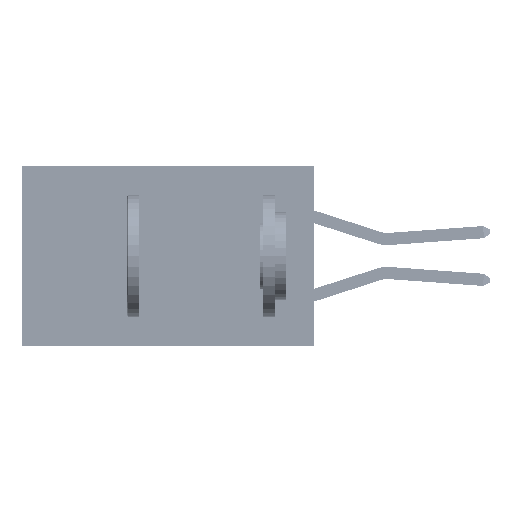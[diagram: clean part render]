
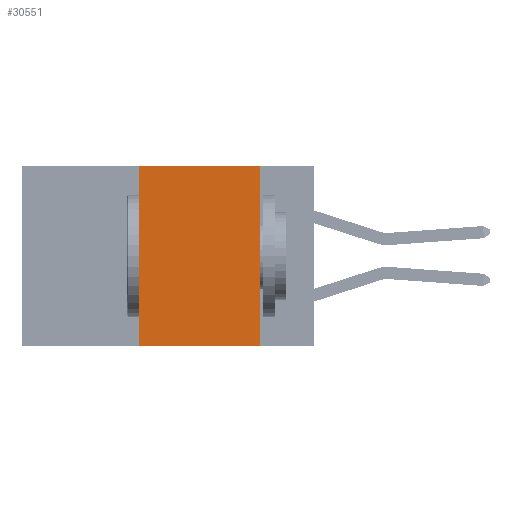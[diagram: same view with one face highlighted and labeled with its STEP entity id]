
A CAD part, left-side view. The second image highlights one B-rep face of the part: STEP entity #30551.
In plain terms, the highlighted planar face has unit normal (-1, 0, 0).
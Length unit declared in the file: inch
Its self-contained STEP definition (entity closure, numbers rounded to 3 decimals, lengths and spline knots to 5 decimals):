
#1260 = VECTOR ( 'NONE', #45532, 39.37008 ) ;
#5038 = CARTESIAN_POINT ( 'NONE',  ( 0., 0.11, 0. ) ) ;
#5152 = ORIENTED_EDGE ( 'NONE', *, *, #28392, .F. ) ;
#5831 = ORIENTED_EDGE ( 'NONE', *, *, #29548, .F. ) ;
#6584 = VECTOR ( 'NONE', #47407, 39.37008 ) ;
#8929 = CARTESIAN_POINT ( 'NONE',  ( 0., 0.36, 0. ) ) ;
#11701 = VERTEX_POINT ( 'NONE', #17921 ) ;
#12452 = EDGE_LOOP ( 'NONE', ( #28630, #5152, #5831, #37780 ) ) ;
#14722 = FACE_OUTER_BOUND ( 'NONE', #12452, .T. ) ;
#15521 = CARTESIAN_POINT ( 'NONE',  ( 0., 0.6, -0.37 ) ) ;
#16817 = LINE ( 'NONE', #29601, #29805 ) ;
#17921 = CARTESIAN_POINT ( 'NONE',  ( 0., 0.11, -0.37 ) ) ;
#18658 = EDGE_CURVE ( 'NONE', #45136, #11701, #45313, .T. ) ;
#19609 = LINE ( 'NONE', #15521, #6584 ) ;
#19800 = LINE ( 'NONE', #8929, #21697 ) ;
#20697 = DIRECTION ( 'NONE',  ( 0., 0., 1. ) ) ;
#21697 = VECTOR ( 'NONE', #20697, 39.37008 ) ;
#23376 = CARTESIAN_POINT ( 'NONE',  ( 0., 0.6, 0. ) ) ;
#26598 = CARTESIAN_POINT ( 'NONE',  ( 0., 0.36, 0. ) ) ;
#28392 = EDGE_CURVE ( 'NONE', #43135, #45136, #16817, .T. ) ;
#28630 = ORIENTED_EDGE ( 'NONE', *, *, #18658, .F. ) ;
#29548 = EDGE_CURVE ( 'NONE', #47060, #43135, #19800, .T. ) ;
#29601 = CARTESIAN_POINT ( 'NONE',  ( 0., 0.6, 0. ) ) ;
#29805 = VECTOR ( 'NONE', #33605, 39.37008 ) ;
#30551 = ADVANCED_FACE ( 'NONE', ( #14722 ), #46959, .F. ) ;
#33561 = CARTESIAN_POINT ( 'NONE',  ( 0., 0.11, 0. ) ) ;
#33605 = DIRECTION ( 'NONE',  ( 0., -1., 0. ) ) ;
#37780 = ORIENTED_EDGE ( 'NONE', *, *, #39767, .T. ) ;
#39767 = EDGE_CURVE ( 'NONE', #47060, #11701, #19609, .T. ) ;
#41378 = AXIS2_PLACEMENT_3D ( 'NONE', #23376, #43492, #46071 ) ;
#41627 = CARTESIAN_POINT ( 'NONE',  ( 0., 0.36, -0.37 ) ) ;
#43135 = VERTEX_POINT ( 'NONE', #26598 ) ;
#43492 = DIRECTION ( 'NONE',  ( 1., 0., 0. ) ) ;
#45136 = VERTEX_POINT ( 'NONE', #5038 ) ;
#45313 = LINE ( 'NONE', #33561, #1260 ) ;
#45532 = DIRECTION ( 'NONE',  ( 0., 0., -1. ) ) ;
#46071 = DIRECTION ( 'NONE',  ( 0., 0., -1. ) ) ;
#46959 = PLANE ( 'NONE',  #41378 ) ;
#47060 = VERTEX_POINT ( 'NONE', #41627 ) ;
#47407 = DIRECTION ( 'NONE',  ( 0., -1., 0. ) ) ;
